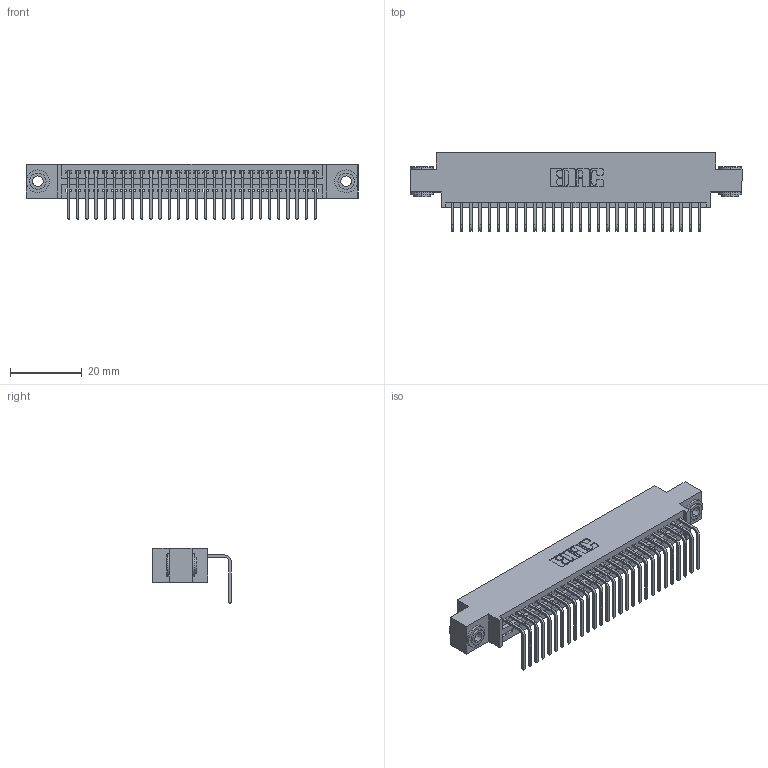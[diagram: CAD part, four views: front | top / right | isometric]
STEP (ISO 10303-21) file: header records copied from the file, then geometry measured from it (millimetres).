
FILE_DESCRIPTION (( 'STEP AP203' ), '1' );
FILE_NAME ('395-028-558-603.STEP', '2019-10-11T05:44:07', ( '' ), ( '' ), 'SwSTEP 2.0', 'SolidWorks 2016', '' );
FILE_SCHEMA (( 'CONFIG_CONTROL_DESIGN' ));
Length unit declared in the file: inch
Products named in the file (4): 345 Part_0.170 Offset - 0.156 Dia-TH; 345-292-001_558 Tail - 2; 345-250-002_345-250-002-102; 395-028-558-603
Assembly tree (31 placements, depth 2):
  395-028-558-603
    345 Part_0.170 Offset - 0.156 Dia-TH
    345-292-001_558 Tail - 2  x28
    345-250-002_345-250-002-102  x2
Bounding box: 92.33 x 21.83 x 15.37 mm (x, y, z)
Volume: 8654.1 mm3; surface area: 12199.5 mm2
Topology: 31 solids, 31 shells, 1848 faces, 5525 edges, 3642 vertices
Faces by surface type: plane 1270, cylinder 570, cone 8
Entity records: 23824 total; most frequent: CARTESIAN_POINT 4107, ORIENTED_EDGE 4062, DIRECTION 3637, EDGE_CURVE 2031, LINE 1763, VECTOR 1763, VERTEX_POINT 1350, AXIS2_PLACEMENT_3D 937
